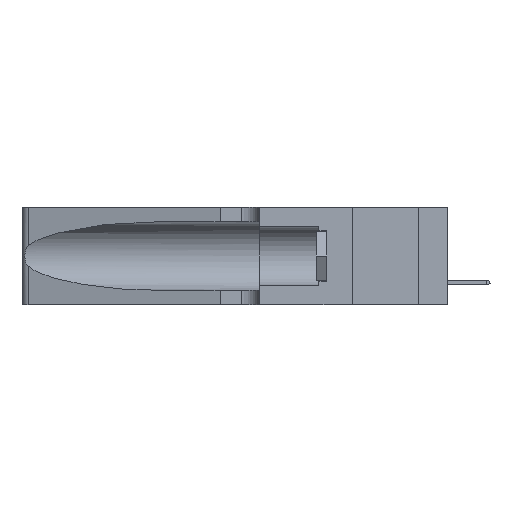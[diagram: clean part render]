
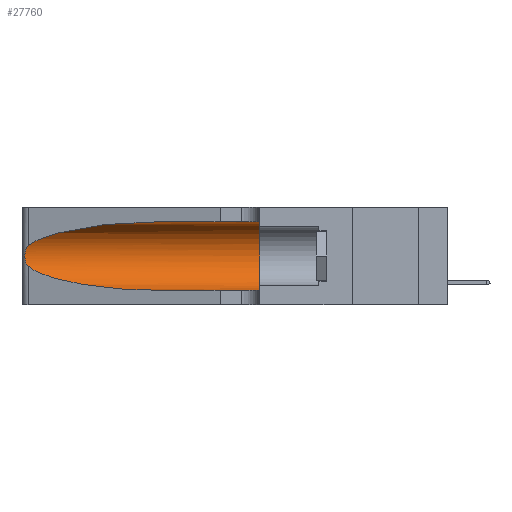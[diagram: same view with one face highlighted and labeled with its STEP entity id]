
A CAD part, left-side view. The second image highlights one B-rep face of the part: STEP entity #27760.
In plain terms, the highlighted cylindrical face has radius 3.308 mm (diameter 6.617 mm), a partial arc.
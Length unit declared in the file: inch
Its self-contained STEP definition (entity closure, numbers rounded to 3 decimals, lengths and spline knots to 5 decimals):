
#1931 = ORIENTED_EDGE ( 'NONE', *, *, #26341, .T. ) ;
#3236 = CARTESIAN_POINT ( 'NONE',  ( 0.25856, 1.23593, 0.16098 ) ) ;
#3542 = CARTESIAN_POINT ( 'NONE',  ( 0.25487, 1.22718, 0.22369 ) ) ;
#4845 = ORIENTED_EDGE ( 'NONE', *, *, #9237, .F. ) ;
#5127 = ORIENTED_EDGE ( 'NONE', *, *, #11494, .F. ) ;
#5734 = FACE_OUTER_BOUND ( 'NONE', #21914, .T. ) ;
#5790 = VERTEX_POINT ( 'NONE', #3542 ) ;
#6165 = CARTESIAN_POINT ( 'NONE',  ( 0.25487, 1.22718, 0.14631 ) ) ;
#6225 = CARTESIAN_POINT ( 'NONE',  ( 0.26075, 1.23896, 0.19203 ) ) ;
#7065 = DIRECTION ( 'NONE',  ( 0., -1., 0. ) ) ;
#7281 = CARTESIAN_POINT ( 'NONE',  ( 0.1305, 0.72297, 0.05475 ) ) ;
#8900 = CARTESIAN_POINT ( 'NONE',  ( 0.25639, 1.23186, 0.15144 ) ) ;
#9000 = CARTESIAN_POINT ( 'NONE',  ( 0.25487, 1.22718, 0.14631 ) ) ;
#9237 = EDGE_CURVE ( 'NONE', #11200, #20312, #26546, .T. ) ;
#10813 = AXIS2_PLACEMENT_3D ( 'NONE', #32099, #23810, #19358 ) ;
#11200 = VERTEX_POINT ( 'NONE', #24967 ) ;
#11286 = CARTESIAN_POINT ( 'NONE',  ( 0.25555, 1.22993, 0.14849 ) ) ;
#11396 = CARTESIAN_POINT ( 'NONE',  ( 0.26018, 1.23835, 0.19895 ) ) ;
#11494 = EDGE_CURVE ( 'NONE', #20312, #12350, #29605, .T. ) ;
#11875 = AXIS2_PLACEMENT_3D ( 'NONE', #33388, #30788, #28007 ) ;
#12309 = LINE ( 'NONE', #33342, #18088 ) ;
#12350 = VERTEX_POINT ( 'NONE', #21633 ) ;
#12588 = VECTOR ( 'NONE', #16903, 39.37008 ) ;
#13955 =( BOUNDED_CURVE ( )  B_SPLINE_CURVE ( 3, ( #6165, #14226, #29880, #15343 ),
 .UNSPECIFIED., .F., .F. ) 
 B_SPLINE_CURVE_WITH_KNOTS ( ( 4, 4 ),
 ( 3.44316, 4.71239 ),
 .UNSPECIFIED. ) 
 CURVE ( )  GEOMETRIC_REPRESENTATION_ITEM ( )  RATIONAL_B_SPLINE_CURVE ( ( 1., 0.87, 0.87, 1. ) ) 
 REPRESENTATION_ITEM ( '' )  );
#14167 = CARTESIAN_POINT ( 'NONE',  ( 0.25487, 1.22718, 0.14631 ) ) ;
#14226 = CARTESIAN_POINT ( 'NONE',  ( 0.2373, 1.15595, 0.08982 ) ) ;
#15343 = CARTESIAN_POINT ( 'NONE',  ( 0.1305, 0.72297, 0.05475 ) ) ;
#15467 = ORIENTED_EDGE ( 'NONE', *, *, #26345, .T. ) ;
#16376 = ORIENTED_EDGE ( 'NONE', *, *, #33955, .T. ) ;
#16441 = EDGE_CURVE ( 'NONE', #5790, #16446, #21110, .T. ) ;
#16446 = VERTEX_POINT ( 'NONE', #9000 ) ;
#16903 = DIRECTION ( 'NONE',  ( 0., -1., 0. ) ) ;
#18088 = VECTOR ( 'NONE', #7065, 39.37008 ) ;
#18666 = CARTESIAN_POINT ( 'NONE',  ( 0.18966, 0.96281, 0.31525 ) ) ;
#19358 = DIRECTION ( 'NONE',  ( 0., 0., -1. ) ) ;
#20312 = VERTEX_POINT ( 'NONE', #21331 ) ;
#21110 = B_SPLINE_CURVE_WITH_KNOTS ( 'NONE', 3,
 ( #24700, #26899, #29812, #24349, #22084, #11396, #6225, #24221, #21849, #3236, #24598, #8900, #11286, #14167 ),
 .UNSPECIFIED., .F., .F.,
 ( 4, 2, 2, 2, 2, 2, 4 ),
 ( 0., 0.00027, 0.00053, 0.00107, 0.0016, 0.00187, 0.00214 ),
 .UNSPECIFIED. ) ;
#21331 = CARTESIAN_POINT ( 'NONE',  ( 0.1305, 0.35, 0.31525 ) ) ;
#21633 = CARTESIAN_POINT ( 'NONE',  ( 0.1305, 0.35, 0.05475 ) ) ;
#21849 = CARTESIAN_POINT ( 'NONE',  ( 0.26017, 1.23833, 0.17102 ) ) ;
#21914 = EDGE_LOOP ( 'NONE', ( #15467, #30523, #1931, #16376, #5127, #4845 ) ) ;
#22025 = CARTESIAN_POINT ( 'NONE',  ( 0.25487, 1.22718, 0.22369 ) ) ;
#22084 = CARTESIAN_POINT ( 'NONE',  ( 0.25854, 1.2359, 0.20912 ) ) ;
#23325 = CARTESIAN_POINT ( 'NONE',  ( 0.2373, 1.15595, 0.28018 ) ) ;
#23781 = CYLINDRICAL_SURFACE ( 'NONE', #10813, 0.13025 ) ;
#23810 = DIRECTION ( 'NONE',  ( 0., -1., 0. ) ) ;
#24221 = CARTESIAN_POINT ( 'NONE',  ( 0.26075, 1.23896, 0.178 ) ) ;
#24349 = CARTESIAN_POINT ( 'NONE',  ( 0.25787, 1.23484, 0.2124 ) ) ;
#24598 = CARTESIAN_POINT ( 'NONE',  ( 0.25789, 1.23486, 0.15765 ) ) ;
#24700 = CARTESIAN_POINT ( 'NONE',  ( 0.25487, 1.22718, 0.22369 ) ) ;
#24967 = CARTESIAN_POINT ( 'NONE',  ( 0.1305, 0.72297, 0.31525 ) ) ;
#26084 = VERTEX_POINT ( 'NONE', #7281 ) ;
#26341 = EDGE_CURVE ( 'NONE', #16446, #26084, #13955, .T. ) ;
#26345 = EDGE_CURVE ( 'NONE', #11200, #5790, #29146, .T. ) ;
#26546 = LINE ( 'NONE', #29914, #12588 ) ;
#26899 = CARTESIAN_POINT ( 'NONE',  ( 0.25555, 1.22994, 0.2215 ) ) ;
#27760 = ADVANCED_FACE ( 'NONE', ( #5734 ), #23781, .F. ) ;
#28007 = DIRECTION ( 'NONE',  ( 0., 0., 1. ) ) ;
#29146 =( BOUNDED_CURVE ( )  B_SPLINE_CURVE ( 3, ( #32586, #18666, #23325, #22025 ),
 .UNSPECIFIED., .F., .T. ) 
 B_SPLINE_CURVE_WITH_KNOTS ( ( 4, 4 ),
 ( 1.5708, 2.84003 ),
 .UNSPECIFIED. ) 
 CURVE ( )  GEOMETRIC_REPRESENTATION_ITEM ( )  RATIONAL_B_SPLINE_CURVE ( ( 1., 0.87, 0.87, 1. ) ) 
 REPRESENTATION_ITEM ( '' )  );
#29605 = CIRCLE ( 'NONE', #11875, 0.13025 ) ;
#29812 = CARTESIAN_POINT ( 'NONE',  ( 0.25639, 1.23184, 0.21858 ) ) ;
#29880 = CARTESIAN_POINT ( 'NONE',  ( 0.18966, 0.96281, 0.05475 ) ) ;
#29914 = CARTESIAN_POINT ( 'NONE',  ( 0.1305, 1.61858, 0.31525 ) ) ;
#30523 = ORIENTED_EDGE ( 'NONE', *, *, #16441, .T. ) ;
#30788 = DIRECTION ( 'NONE',  ( 0., 1., 0. ) ) ;
#32099 = CARTESIAN_POINT ( 'NONE',  ( 0.1305, 1.61858, 0.185 ) ) ;
#32586 = CARTESIAN_POINT ( 'NONE',  ( 0.1305, 0.72297, 0.31525 ) ) ;
#33342 = CARTESIAN_POINT ( 'NONE',  ( 0.1305, 1.61858, 0.05475 ) ) ;
#33388 = CARTESIAN_POINT ( 'NONE',  ( 0.1305, 0.35, 0.185 ) ) ;
#33955 = EDGE_CURVE ( 'NONE', #26084, #12350, #12309, .T. ) ;
